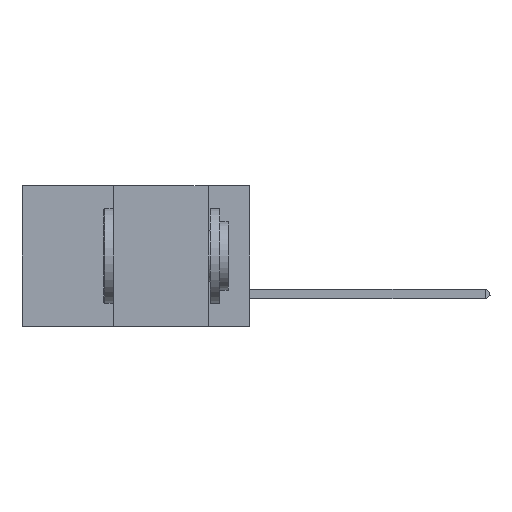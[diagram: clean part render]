
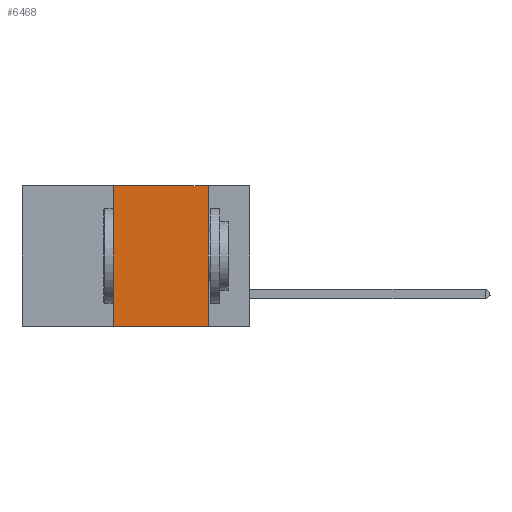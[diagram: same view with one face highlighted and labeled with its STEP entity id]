
A CAD part, left-side view. The second image highlights one B-rep face of the part: STEP entity #6468.
In plain terms, the highlighted planar face has unit normal (-1, 0, 0).
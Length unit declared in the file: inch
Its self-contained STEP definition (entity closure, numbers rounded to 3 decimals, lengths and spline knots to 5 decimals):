
#428 = LINE ( 'NONE', #25438, #4257 ) ;
#602 = DIRECTION ( 'NONE',  ( 1., 0., 0. ) ) ;
#1018 = CARTESIAN_POINT ( 'NONE',  ( 0., 0.11, -0.37 ) ) ;
#1410 = VECTOR ( 'NONE', #18181, 39.37008 ) ;
#1923 = ORIENTED_EDGE ( 'NONE', *, *, #3644, .F. ) ;
#3644 = EDGE_CURVE ( 'NONE', #13951, #16930, #11772, .T. ) ;
#4257 = VECTOR ( 'NONE', #7042, 39.37008 ) ;
#4786 = LINE ( 'NONE', #15619, #19688 ) ;
#5133 = AXIS2_PLACEMENT_3D ( 'NONE', #14771, #602, #8789 ) ;
#6468 = ADVANCED_FACE ( 'NONE', ( #16680 ), #6722, .F. ) ;
#6722 = PLANE ( 'NONE',  #5133 ) ;
#6822 = DIRECTION ( 'NONE',  ( 0., 0., -1. ) ) ;
#7042 = DIRECTION ( 'NONE',  ( 0., 0., 1. ) ) ;
#7854 = CARTESIAN_POINT ( 'NONE',  ( 0., 0.11, 0. ) ) ;
#8789 = DIRECTION ( 'NONE',  ( 0., 0., -1. ) ) ;
#10026 = LINE ( 'NONE', #22152, #1410 ) ;
#11772 = LINE ( 'NONE', #24622, #17162 ) ;
#12054 = EDGE_CURVE ( 'NONE', #21908, #16930, #10026, .T. ) ;
#12867 = ORIENTED_EDGE ( 'NONE', *, *, #12054, .T. ) ;
#12876 = EDGE_CURVE ( 'NONE', #21908, #20501, #428, .T. ) ;
#13951 = VERTEX_POINT ( 'NONE', #7854 ) ;
#14404 = ORIENTED_EDGE ( 'NONE', *, *, #12876, .F. ) ;
#14568 = EDGE_CURVE ( 'NONE', #20501, #13951, #4786, .T. ) ;
#14771 = CARTESIAN_POINT ( 'NONE',  ( 0., 0.6, 0. ) ) ;
#15027 = CARTESIAN_POINT ( 'NONE',  ( 0., 0.36, -0.37 ) ) ;
#15619 = CARTESIAN_POINT ( 'NONE',  ( 0., 0.6, 0. ) ) ;
#16596 = CARTESIAN_POINT ( 'NONE',  ( 0., 0.36, 0. ) ) ;
#16680 = FACE_OUTER_BOUND ( 'NONE', #18578, .T. ) ;
#16930 = VERTEX_POINT ( 'NONE', #1018 ) ;
#17162 = VECTOR ( 'NONE', #6822, 39.37008 ) ;
#17956 = ORIENTED_EDGE ( 'NONE', *, *, #14568, .F. ) ;
#18181 = DIRECTION ( 'NONE',  ( 0., -1., 0. ) ) ;
#18578 = EDGE_LOOP ( 'NONE', ( #1923, #17956, #14404, #12867 ) ) ;
#19688 = VECTOR ( 'NONE', #23336, 39.37008 ) ;
#20501 = VERTEX_POINT ( 'NONE', #16596 ) ;
#21908 = VERTEX_POINT ( 'NONE', #15027 ) ;
#22152 = CARTESIAN_POINT ( 'NONE',  ( 0., 0.6, -0.37 ) ) ;
#23336 = DIRECTION ( 'NONE',  ( 0., -1., 0. ) ) ;
#24622 = CARTESIAN_POINT ( 'NONE',  ( 0., 0.11, 0. ) ) ;
#25438 = CARTESIAN_POINT ( 'NONE',  ( 0., 0.36, 0. ) ) ;
